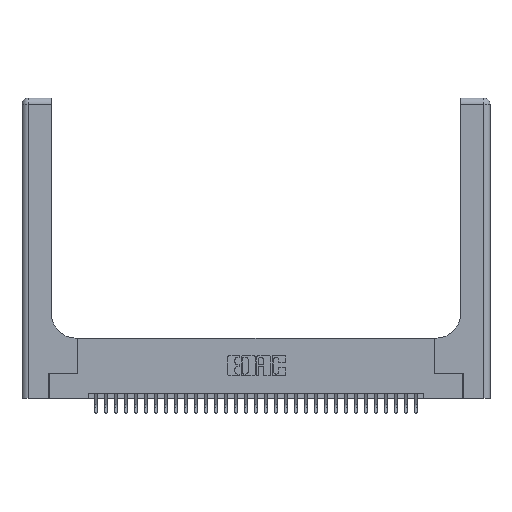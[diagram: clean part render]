
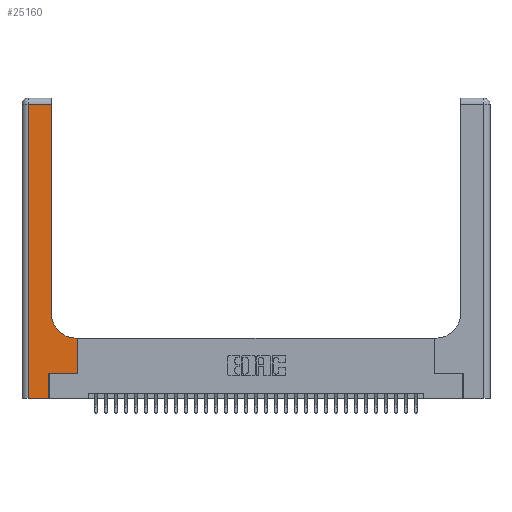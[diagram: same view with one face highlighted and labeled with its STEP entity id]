
A CAD part, top view. The second image highlights one B-rep face of the part: STEP entity #25160.
In plain terms, the highlighted planar face has unit normal (0, 0, 1).
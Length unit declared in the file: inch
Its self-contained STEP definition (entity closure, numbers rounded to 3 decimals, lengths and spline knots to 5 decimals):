
#909 = EDGE_CURVE ( 'NONE', #31488, #6418, #24438, .T. ) ;
#968 = ORIENTED_EDGE ( 'NONE', *, *, #24363, .T. ) ;
#1279 = CARTESIAN_POINT ( 'NONE',  ( 0., 2.94, 0.37 ) ) ;
#1568 = CARTESIAN_POINT ( 'NONE',  ( 0.5585, 0.6, 0.37 ) ) ;
#4058 = LINE ( 'NONE', #27216, #21750 ) ;
#4556 = EDGE_CURVE ( 'NONE', #28082, #21843, #18357, .T. ) ;
#5115 = ORIENTED_EDGE ( 'NONE', *, *, #15537, .T. ) ;
#5383 = EDGE_CURVE ( 'NONE', #18034, #31488, #8056, .T. ) ;
#6043 = CARTESIAN_POINT ( 'NONE',  ( 0.06, 3., 0.37 ) ) ;
#6418 = VERTEX_POINT ( 'NONE', #19231 ) ;
#6421 = PLANE ( 'NONE',  #12552 ) ;
#6581 = DIRECTION ( 'NONE',  ( 0., 1., 0. ) ) ;
#7040 = EDGE_CURVE ( 'NONE', #6418, #18944, #21189, .T. ) ;
#7453 = DIRECTION ( 'NONE',  ( 0., 1., 0. ) ) ;
#7942 = CARTESIAN_POINT ( 'NONE',  ( 0.2915, 0.85, 0.37 ) ) ;
#8056 = LINE ( 'NONE', #8689, #28886 ) ;
#8242 = CARTESIAN_POINT ( 'NONE',  ( 0.269, 0.25, 0.37 ) ) ;
#8689 = CARTESIAN_POINT ( 'NONE',  ( 0.5585, 0.25, 0.37 ) ) ;
#8982 = DIRECTION ( 'NONE',  ( -1., 0., 0. ) ) ;
#9275 = LINE ( 'NONE', #8242, #14403 ) ;
#9424 = EDGE_CURVE ( 'NONE', #17193, #18034, #9275, .T. ) ;
#9745 = VERTEX_POINT ( 'NONE', #27206 ) ;
#9879 = ORIENTED_EDGE ( 'NONE', *, *, #12751, .T. ) ;
#10888 = EDGE_CURVE ( 'NONE', #13281, #28082, #19374, .T. ) ;
#11029 = DIRECTION ( 'NONE',  ( -1., 0., 0. ) ) ;
#11635 = CARTESIAN_POINT ( 'NONE',  ( 0.06, 0., 0.37 ) ) ;
#11672 = DIRECTION ( 'NONE',  ( 1., 0., 0. ) ) ;
#11998 = ORIENTED_EDGE ( 'NONE', *, *, #10888, .T. ) ;
#12162 = FACE_OUTER_BOUND ( 'NONE', #21726, .T. ) ;
#12552 = AXIS2_PLACEMENT_3D ( 'NONE', #24014, #26641, #8982 ) ;
#12751 = EDGE_CURVE ( 'NONE', #21843, #17193, #4058, .T. ) ;
#13281 = VERTEX_POINT ( 'NONE', #18784 ) ;
#13812 = CARTESIAN_POINT ( 'NONE',  ( 0.269, 0.25, 0.37 ) ) ;
#14403 = VECTOR ( 'NONE', #21105, 39.37008 ) ;
#14407 = CARTESIAN_POINT ( 'NONE',  ( 0.5585, 0.25, 0.37 ) ) ;
#14621 = CARTESIAN_POINT ( 'NONE',  ( 0.2915, 0.6, 0.37 ) ) ;
#15054 = VECTOR ( 'NONE', #24694, 39.37008 ) ;
#15537 = EDGE_CURVE ( 'NONE', #9745, #13281, #17640, .T. ) ;
#15637 = VECTOR ( 'NONE', #20182, 39.37008 ) ;
#15855 = ORIENTED_EDGE ( 'NONE', *, *, #5383, .T. ) ;
#17170 = DIRECTION ( 'NONE',  ( 0., 1., 0. ) ) ;
#17193 = VERTEX_POINT ( 'NONE', #13812 ) ;
#17517 = CARTESIAN_POINT ( 'NONE',  ( 0.269, 0., 0.37 ) ) ;
#17640 = LINE ( 'NONE', #1279, #27017 ) ;
#18034 = VERTEX_POINT ( 'NONE', #14407 ) ;
#18357 = LINE ( 'NONE', #22582, #15637 ) ;
#18784 = CARTESIAN_POINT ( 'NONE',  ( 0.06, 2.94, 0.37 ) ) ;
#18944 = VERTEX_POINT ( 'NONE', #7942 ) ;
#18966 = CARTESIAN_POINT ( 'NONE',  ( 0.5415, 0.85, 0.37 ) ) ;
#19231 = CARTESIAN_POINT ( 'NONE',  ( 0.5415, 0.6, 0.37 ) ) ;
#19251 = CARTESIAN_POINT ( 'NONE',  ( 0.2915, 3., 0.37 ) ) ;
#19374 = LINE ( 'NONE', #6043, #24073 ) ;
#20182 = DIRECTION ( 'NONE',  ( 1., 0., 0. ) ) ;
#21105 = DIRECTION ( 'NONE',  ( 1., 0., 0. ) ) ;
#21189 = CIRCLE ( 'NONE', #32073, 0.25 ) ;
#21726 = EDGE_LOOP ( 'NONE', ( #968, #5115, #11998, #27346, #9879, #27991, #15855, #32421, #29324 ) ) ;
#21750 = VECTOR ( 'NONE', #7453, 39.37008 ) ;
#21843 = VERTEX_POINT ( 'NONE', #17517 ) ;
#22582 = CARTESIAN_POINT ( 'NONE',  ( 0., 0., 0.37 ) ) ;
#23965 = DIRECTION ( 'NONE',  ( 0., -1., 0. ) ) ;
#23996 = DIRECTION ( 'NONE',  ( 0., 0., -1. ) ) ;
#24014 = CARTESIAN_POINT ( 'NONE',  ( 0., 3., 0.37 ) ) ;
#24073 = VECTOR ( 'NONE', #23965, 39.37008 ) ;
#24363 = EDGE_CURVE ( 'NONE', #18944, #9745, #29904, .T. ) ;
#24438 = LINE ( 'NONE', #14621, #15054 ) ;
#24694 = DIRECTION ( 'NONE',  ( -1., 0., 0. ) ) ;
#25160 = ADVANCED_FACE ( 'NONE', ( #12162 ), #6421, .F. ) ;
#26349 = VECTOR ( 'NONE', #6581, 39.37008 ) ;
#26641 = DIRECTION ( 'NONE',  ( 0., 0., -1. ) ) ;
#27017 = VECTOR ( 'NONE', #11029, 39.37008 ) ;
#27206 = CARTESIAN_POINT ( 'NONE',  ( 0.2915, 2.94, 0.37 ) ) ;
#27216 = CARTESIAN_POINT ( 'NONE',  ( 0.269, 0., 0.37 ) ) ;
#27346 = ORIENTED_EDGE ( 'NONE', *, *, #4556, .T. ) ;
#27991 = ORIENTED_EDGE ( 'NONE', *, *, #9424, .T. ) ;
#28082 = VERTEX_POINT ( 'NONE', #11635 ) ;
#28886 = VECTOR ( 'NONE', #17170, 39.37008 ) ;
#29324 = ORIENTED_EDGE ( 'NONE', *, *, #7040, .T. ) ;
#29904 = LINE ( 'NONE', #19251, #26349 ) ;
#31488 = VERTEX_POINT ( 'NONE', #1568 ) ;
#32073 = AXIS2_PLACEMENT_3D ( 'NONE', #18966, #23996, #11672 ) ;
#32421 = ORIENTED_EDGE ( 'NONE', *, *, #909, .T. ) ;
